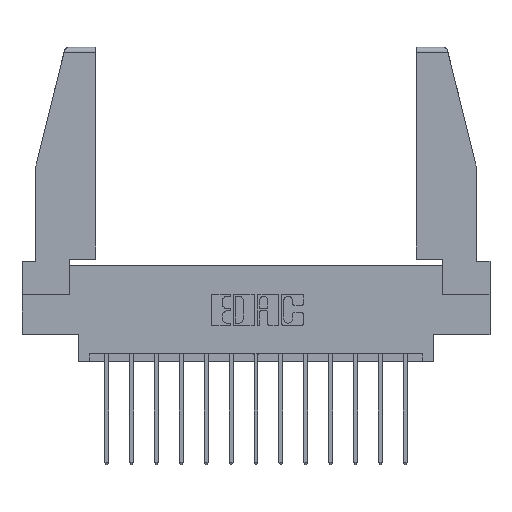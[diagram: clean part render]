
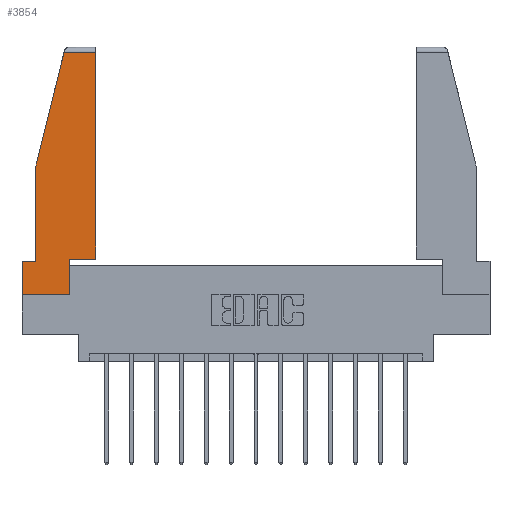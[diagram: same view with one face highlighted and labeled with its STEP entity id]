
A CAD part, top view. The second image highlights one B-rep face of the part: STEP entity #3854.
In plain terms, the highlighted planar face has unit normal (0, 0, 1).
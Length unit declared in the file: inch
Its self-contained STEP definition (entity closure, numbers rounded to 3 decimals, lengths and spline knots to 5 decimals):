
#416 = DIRECTION ( 'NONE',  ( 0., -1., 0. ) ) ;
#552 = VECTOR ( 'NONE', #13202, 39.37008 ) ;
#625 = VERTEX_POINT ( 'NONE', #8820 ) ;
#666 = LINE ( 'NONE', #15758, #6798 ) ;
#839 = CARTESIAN_POINT ( 'NONE',  ( 0.271, 1.55, 0. ) ) ;
#958 = EDGE_CURVE ( 'NONE', #12516, #7887, #666, .T. ) ;
#969 = ORIENTED_EDGE ( 'NONE', *, *, #11018, .T. ) ;
#1235 = VECTOR ( 'NONE', #11130, 39.37008 ) ;
#1277 = EDGE_CURVE ( 'NONE', #625, #15885, #5010, .T. ) ;
#1526 = ORIENTED_EDGE ( 'NONE', *, *, #2531, .T. ) ;
#1768 = LINE ( 'NONE', #5319, #9503 ) ;
#1925 = EDGE_LOOP ( 'NONE', ( #13559, #13005, #12721, #8316, #969, #3957, #10642, #1526, #7944 ) ) ;
#2531 = EDGE_CURVE ( 'NONE', #6126, #3599, #11442, .T. ) ;
#2627 = VECTOR ( 'NONE', #4700, 39.37008 ) ;
#2742 = LINE ( 'NONE', #9843, #15879 ) ;
#3301 = CARTESIAN_POINT ( 'NONE',  ( 0., 0.21, 0. ) ) ;
#3562 = VERTEX_POINT ( 'NONE', #13214 ) ;
#3599 = VERTEX_POINT ( 'NONE', #15802 ) ;
#3692 = DIRECTION ( 'NONE',  ( 0., 0., 1. ) ) ;
#3854 = ADVANCED_FACE ( 'NONE', ( #7032 ), #15049, .T. ) ;
#3957 = ORIENTED_EDGE ( 'NONE', *, *, #1277, .T. ) ;
#4700 = DIRECTION ( 'NONE',  ( 1., 0., 0. ) ) ;
#4960 = EDGE_CURVE ( 'NONE', #3599, #13589, #9190, .T. ) ;
#5010 = LINE ( 'NONE', #12878, #9184 ) ;
#5017 = DIRECTION ( 'NONE',  ( 1., 0., 0. ) ) ;
#5222 = LINE ( 'NONE', #10971, #2627 ) ;
#5319 = CARTESIAN_POINT ( 'NONE',  ( 0.461, 0.223, 0. ) ) ;
#5659 = VECTOR ( 'NONE', #13460, 39.37008 ) ;
#5750 = EDGE_CURVE ( 'NONE', #15885, #6126, #5222, .T. ) ;
#6061 = DIRECTION ( 'NONE',  ( -1., 0., 0. ) ) ;
#6126 = VERTEX_POINT ( 'NONE', #10454 ) ;
#6224 = CARTESIAN_POINT ( 'NONE',  ( 0., 0., 0. ) ) ;
#6227 = DIRECTION ( 'NONE',  ( 1., 0., 0. ) ) ;
#6444 = DIRECTION ( 'NONE',  ( 0., -1., 0. ) ) ;
#6798 = VECTOR ( 'NONE', #6444, 39.37008 ) ;
#7032 = FACE_OUTER_BOUND ( 'NONE', #1925, .T. ) ;
#7887 = VERTEX_POINT ( 'NONE', #9750 ) ;
#7944 = ORIENTED_EDGE ( 'NONE', *, *, #4960, .T. ) ;
#8316 = ORIENTED_EDGE ( 'NONE', *, *, #958, .T. ) ;
#8317 = DIRECTION ( 'NONE',  ( 0., 1., 0. ) ) ;
#8739 = CARTESIAN_POINT ( 'NONE',  ( 0.297, 0.223, 0. ) ) ;
#8820 = CARTESIAN_POINT ( 'NONE',  ( 0., 0.21, 0. ) ) ;
#9183 = LINE ( 'NONE', #3301, #1235 ) ;
#9184 = VECTOR ( 'NONE', #416, 39.37008 ) ;
#9190 = LINE ( 'NONE', #8739, #14557 ) ;
#9384 = EDGE_CURVE ( 'NONE', #9479, #12516, #15603, .T. ) ;
#9479 = VERTEX_POINT ( 'NONE', #14866 ) ;
#9503 = VECTOR ( 'NONE', #8317, 39.37008 ) ;
#9750 = CARTESIAN_POINT ( 'NONE',  ( 0.086, 0.21, 0. ) ) ;
#9843 = CARTESIAN_POINT ( 'NONE',  ( 0., 1.52, 0. ) ) ;
#10378 = CARTESIAN_POINT ( 'NONE',  ( 0.461, 0.223, 0. ) ) ;
#10454 = CARTESIAN_POINT ( 'NONE',  ( 0.297, 0., 0. ) ) ;
#10642 = ORIENTED_EDGE ( 'NONE', *, *, #5750, .T. ) ;
#10971 = CARTESIAN_POINT ( 'NONE',  ( 0., 0., 0. ) ) ;
#11018 = EDGE_CURVE ( 'NONE', #7887, #625, #9183, .T. ) ;
#11130 = DIRECTION ( 'NONE',  ( -1., 0., 0. ) ) ;
#11200 = AXIS2_PLACEMENT_3D ( 'NONE', #6224, #3692, #5017 ) ;
#11442 = LINE ( 'NONE', #14448, #552 ) ;
#12516 = VERTEX_POINT ( 'NONE', #15031 ) ;
#12721 = ORIENTED_EDGE ( 'NONE', *, *, #9384, .T. ) ;
#12878 = CARTESIAN_POINT ( 'NONE',  ( 0., 0.21, 0. ) ) ;
#13005 = ORIENTED_EDGE ( 'NONE', *, *, #13300, .T. ) ;
#13202 = DIRECTION ( 'NONE',  ( 0., 1., 0. ) ) ;
#13214 = CARTESIAN_POINT ( 'NONE',  ( 0.461, 1.52, 0. ) ) ;
#13300 = EDGE_CURVE ( 'NONE', #3562, #9479, #2742, .T. ) ;
#13460 = DIRECTION ( 'NONE',  ( -0.239, -0.971, 0. ) ) ;
#13559 = ORIENTED_EDGE ( 'NONE', *, *, #14846, .T. ) ;
#13589 = VERTEX_POINT ( 'NONE', #10378 ) ;
#14448 = CARTESIAN_POINT ( 'NONE',  ( 0.297, 0., 0. ) ) ;
#14557 = VECTOR ( 'NONE', #6227, 39.37008 ) ;
#14846 = EDGE_CURVE ( 'NONE', #13589, #3562, #1768, .T. ) ;
#14866 = CARTESIAN_POINT ( 'NONE',  ( 0.2636, 1.52, 0. ) ) ;
#15031 = CARTESIAN_POINT ( 'NONE',  ( 0.086, 0.8, 0. ) ) ;
#15049 = PLANE ( 'NONE',  #11200 ) ;
#15603 = LINE ( 'NONE', #839, #5659 ) ;
#15758 = CARTESIAN_POINT ( 'NONE',  ( 0.086, 0.8, 0. ) ) ;
#15797 = CARTESIAN_POINT ( 'NONE',  ( 0., 0., 0. ) ) ;
#15802 = CARTESIAN_POINT ( 'NONE',  ( 0.297, 0.223, 0. ) ) ;
#15879 = VECTOR ( 'NONE', #6061, 39.37008 ) ;
#15885 = VERTEX_POINT ( 'NONE', #15797 ) ;
